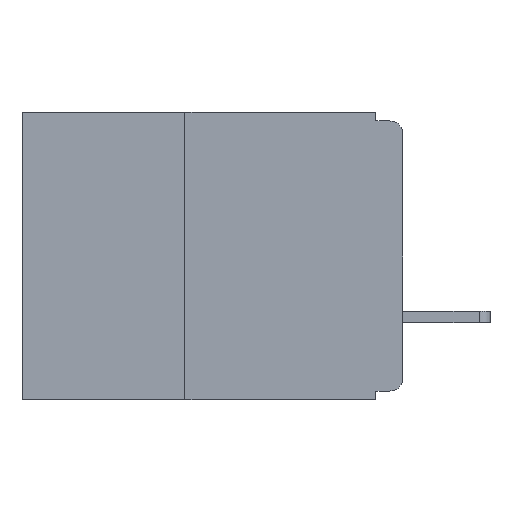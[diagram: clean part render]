
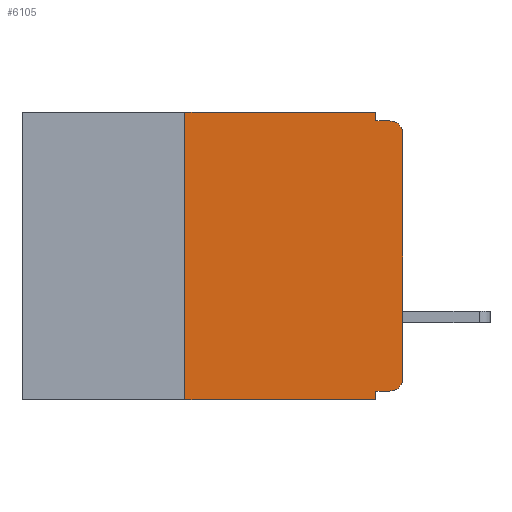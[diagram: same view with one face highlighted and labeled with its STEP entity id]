
A CAD part, left-side view. The second image highlights one B-rep face of the part: STEP entity #6105.
In plain terms, the highlighted planar face has unit normal (-1, 0, 0).
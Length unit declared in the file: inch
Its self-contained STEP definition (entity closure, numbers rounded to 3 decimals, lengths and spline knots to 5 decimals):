
#1403 = DIRECTION ( 'NONE',  ( 0., 0., -1. ) ) ;
#1428 = ORIENTED_EDGE ( 'NONE', *, *, #2039, .T. ) ;
#1440 = CARTESIAN_POINT ( 'NONE',  ( 0., 0.031, 0. ) ) ;
#2039 = EDGE_CURVE ( 'NONE', #2512, #3155, #2190, .T. ) ;
#2167 = EDGE_CURVE ( 'NONE', #11853, #14124, #15823, .T. ) ;
#2190 = CIRCLE ( 'NONE', #13118, 0.015 ) ;
#2450 = EDGE_CURVE ( 'NONE', #6662, #11853, #9630, .T. ) ;
#2512 = VERTEX_POINT ( 'NONE', #3110 ) ;
#2645 = EDGE_LOOP ( 'NONE', ( #3364, #1428, #5084, #7159, #9920, #3991, #16187, #16809, #17415, #11773 ) ) ;
#3110 = CARTESIAN_POINT ( 'NONE',  ( 0., 0., -0.025 ) ) ;
#3155 = VERTEX_POINT ( 'NONE', #3926 ) ;
#3306 = DIRECTION ( 'NONE',  ( 0., 0., 1. ) ) ;
#3364 = ORIENTED_EDGE ( 'NONE', *, *, #17857, .T. ) ;
#3429 = CARTESIAN_POINT ( 'NONE',  ( 0., 0.437, -0.33 ) ) ;
#3770 = DIRECTION ( 'NONE',  ( 0., 0., -1. ) ) ;
#3792 = DIRECTION ( 'NONE',  ( -1., 0., 0. ) ) ;
#3843 = CARTESIAN_POINT ( 'NONE',  ( 0., 0.015, -0.305 ) ) ;
#3926 = CARTESIAN_POINT ( 'NONE',  ( 0., 0.015, -0.01 ) ) ;
#3991 = ORIENTED_EDGE ( 'NONE', *, *, #2450, .F. ) ;
#4259 = DIRECTION ( 'NONE',  ( 0., 0., -1. ) ) ;
#4276 = DIRECTION ( 'NONE',  ( 1., 0., 0. ) ) ;
#4323 = CARTESIAN_POINT ( 'NONE',  ( 0., 0.437, 0. ) ) ;
#4342 = PLANE ( 'NONE',  #8786 ) ;
#4417 = DIRECTION ( 'NONE',  ( 0., 0., -1. ) ) ;
#4431 = EDGE_CURVE ( 'NONE', #13225, #13117, #12457, .T. ) ;
#4652 = VECTOR ( 'NONE', #7806, 39.37008 ) ;
#4691 = VECTOR ( 'NONE', #6811, 39.37008 ) ;
#4843 = VERTEX_POINT ( 'NONE', #16735 ) ;
#4854 = CARTESIAN_POINT ( 'NONE',  ( 0., 0., -0.32 ) ) ;
#5084 = ORIENTED_EDGE ( 'NONE', *, *, #17973, .F. ) ;
#5667 = VECTOR ( 'NONE', #6512, 39.37008 ) ;
#5708 = CARTESIAN_POINT ( 'NONE',  ( 0., 0.015, -0.025 ) ) ;
#5725 = VECTOR ( 'NONE', #6728, 39.37008 ) ;
#5827 = EDGE_CURVE ( 'NONE', #9326, #4843, #9686, .T. ) ;
#6020 = CARTESIAN_POINT ( 'NONE',  ( 0., 0.25, -0.33 ) ) ;
#6105 = ADVANCED_FACE ( 'NONE', ( #12597 ), #4342, .F. ) ;
#6436 = EDGE_CURVE ( 'NONE', #14124, #6976, #18335, .T. ) ;
#6512 = DIRECTION ( 'NONE',  ( 0., 0., 1. ) ) ;
#6662 = VERTEX_POINT ( 'NONE', #13994 ) ;
#6728 = DIRECTION ( 'NONE',  ( 0., 0., -1. ) ) ;
#6811 = DIRECTION ( 'NONE',  ( 0., -1., 0. ) ) ;
#6813 = CARTESIAN_POINT ( 'NONE',  ( 0., 0.031, -0.33 ) ) ;
#6976 = VERTEX_POINT ( 'NONE', #10213 ) ;
#7159 = ORIENTED_EDGE ( 'NONE', *, *, #6436, .F. ) ;
#7293 = VECTOR ( 'NONE', #17705, 39.37008 ) ;
#7806 = DIRECTION ( 'NONE',  ( 0., 1., 0. ) ) ;
#7817 = LINE ( 'NONE', #3429, #18804 ) ;
#8052 = DIRECTION ( 'NONE',  ( -1., 0., 0. ) ) ;
#8578 = LINE ( 'NONE', #4854, #4652 ) ;
#8608 = LINE ( 'NONE', #11328, #4691 ) ;
#8786 = AXIS2_PLACEMENT_3D ( 'NONE', #4323, #4276, #4259 ) ;
#9326 = VERTEX_POINT ( 'NONE', #15988 ) ;
#9479 = CARTESIAN_POINT ( 'NONE',  ( 0., 0.015, -0.32 ) ) ;
#9630 = LINE ( 'NONE', #6020, #5667 ) ;
#9686 = LINE ( 'NONE', #6813, #5725 ) ;
#9920 = ORIENTED_EDGE ( 'NONE', *, *, #2167, .F. ) ;
#10040 = AXIS2_PLACEMENT_3D ( 'NONE', #3843, #3792, #3770 ) ;
#10173 = CARTESIAN_POINT ( 'NONE',  ( 0., 0.031, 0. ) ) ;
#10213 = CARTESIAN_POINT ( 'NONE',  ( 0., 0.031, -0.01 ) ) ;
#11328 = CARTESIAN_POINT ( 'NONE',  ( 0., 0., -0.01 ) ) ;
#11511 = VECTOR ( 'NONE', #3306, 39.37008 ) ;
#11773 = ORIENTED_EDGE ( 'NONE', *, *, #4431, .T. ) ;
#11853 = VERTEX_POINT ( 'NONE', #17119 ) ;
#12342 = CARTESIAN_POINT ( 'NONE',  ( 0., 0., 0. ) ) ;
#12457 = CIRCLE ( 'NONE', #10040, 0.015 ) ;
#12597 = FACE_OUTER_BOUND ( 'NONE', #2645, .T. ) ;
#13117 = VERTEX_POINT ( 'NONE', #13843 ) ;
#13118 = AXIS2_PLACEMENT_3D ( 'NONE', #5708, #8052, #4417 ) ;
#13225 = VERTEX_POINT ( 'NONE', #9479 ) ;
#13773 = EDGE_CURVE ( 'NONE', #13225, #9326, #8578, .T. ) ;
#13843 = CARTESIAN_POINT ( 'NONE',  ( 0., 0., -0.305 ) ) ;
#13981 = VECTOR ( 'NONE', #1403, 39.37008 ) ;
#13994 = CARTESIAN_POINT ( 'NONE',  ( 0., 0.25, -0.33 ) ) ;
#14124 = VERTEX_POINT ( 'NONE', #10173 ) ;
#14932 = EDGE_CURVE ( 'NONE', #6662, #4843, #7817, .T. ) ;
#15823 = LINE ( 'NONE', #17665, #7293 ) ;
#15988 = CARTESIAN_POINT ( 'NONE',  ( 0., 0.031, -0.32 ) ) ;
#16187 = ORIENTED_EDGE ( 'NONE', *, *, #14932, .T. ) ;
#16735 = CARTESIAN_POINT ( 'NONE',  ( 0., 0.031, -0.33 ) ) ;
#16809 = ORIENTED_EDGE ( 'NONE', *, *, #5827, .F. ) ;
#17119 = CARTESIAN_POINT ( 'NONE',  ( 0., 0.25, 0. ) ) ;
#17415 = ORIENTED_EDGE ( 'NONE', *, *, #13773, .F. ) ;
#17665 = CARTESIAN_POINT ( 'NONE',  ( 0., 0.437, 0. ) ) ;
#17705 = DIRECTION ( 'NONE',  ( 0., -1., 0. ) ) ;
#17857 = EDGE_CURVE ( 'NONE', #13117, #2512, #18464, .T. ) ;
#17973 = EDGE_CURVE ( 'NONE', #6976, #3155, #8608, .T. ) ;
#18328 = DIRECTION ( 'NONE',  ( 0., -1., 0. ) ) ;
#18335 = LINE ( 'NONE', #1440, #13981 ) ;
#18464 = LINE ( 'NONE', #12342, #11511 ) ;
#18804 = VECTOR ( 'NONE', #18328, 39.37008 ) ;
